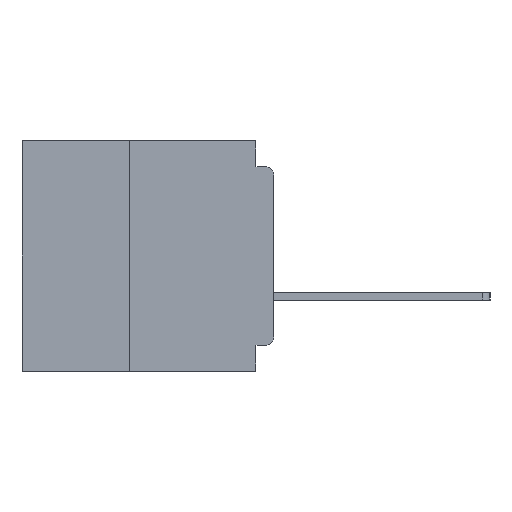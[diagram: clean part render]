
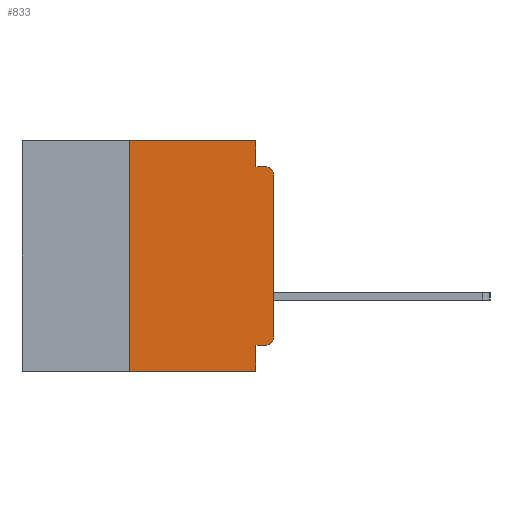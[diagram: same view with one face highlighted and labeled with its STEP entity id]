
A CAD part, left-side view. The second image highlights one B-rep face of the part: STEP entity #833.
In plain terms, the highlighted planar face has unit normal (-1, 0, 0).
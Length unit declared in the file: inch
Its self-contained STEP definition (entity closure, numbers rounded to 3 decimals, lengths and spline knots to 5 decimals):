
#833 = ADVANCED_FACE ( 'NONE', ( #34483 ), #24747, .F. ) ;
#1700 = CARTESIAN_POINT ( 'NONE',  ( 0., 0.25, -0.4 ) ) ;
#1888 = AXIS2_PLACEMENT_3D ( 'NONE', #8199, #30971, #11540 ) ;
#2004 = DIRECTION ( 'NONE',  ( 0., 0., -1. ) ) ;
#3078 = VECTOR ( 'NONE', #28970, 39.37008 ) ;
#3546 = CARTESIAN_POINT ( 'NONE',  ( 0., 0.031, -0.045 ) ) ;
#4341 = EDGE_CURVE ( 'NONE', #12091, #6310, #36215, .T. ) ;
#4519 = AXIS2_PLACEMENT_3D ( 'NONE', #5737, #12362, #33074 ) ;
#4864 = CARTESIAN_POINT ( 'NONE',  ( 0., 0.437, -0.4 ) ) ;
#5737 = CARTESIAN_POINT ( 'NONE',  ( 0., 0.437, 0. ) ) ;
#6036 = LINE ( 'NONE', #22973, #40578 ) ;
#6056 = CARTESIAN_POINT ( 'NONE',  ( 0., 0.437, 0. ) ) ;
#6310 = VERTEX_POINT ( 'NONE', #41696 ) ;
#6541 = DIRECTION ( 'NONE',  ( 0., 0., 1. ) ) ;
#7229 = CARTESIAN_POINT ( 'NONE',  ( 0., 0., -0.06 ) ) ;
#7596 = ORIENTED_EDGE ( 'NONE', *, *, #29237, .F. ) ;
#7837 = CARTESIAN_POINT ( 'NONE',  ( 0., 0.015, -0.045 ) ) ;
#8014 = VERTEX_POINT ( 'NONE', #34835 ) ;
#8199 = CARTESIAN_POINT ( 'NONE',  ( 0., 0.015, -0.06 ) ) ;
#8416 = VERTEX_POINT ( 'NONE', #7837 ) ;
#8813 = EDGE_LOOP ( 'NONE', ( #40553, #31541, #15379, #7596, #10747, #30078, #39593, #16959, #27591, #11272 ) ) ;
#10429 = DIRECTION ( 'NONE',  ( 0., 0., -1. ) ) ;
#10747 = ORIENTED_EDGE ( 'NONE', *, *, #38561, .F. ) ;
#11272 = ORIENTED_EDGE ( 'NONE', *, *, #4341, .T. ) ;
#11540 = DIRECTION ( 'NONE',  ( 0., 0., -1. ) ) ;
#12091 = VERTEX_POINT ( 'NONE', #33267 ) ;
#12362 = DIRECTION ( 'NONE',  ( 1., 0., 0. ) ) ;
#12911 = LINE ( 'NONE', #27486, #37669 ) ;
#13621 = CARTESIAN_POINT ( 'NONE',  ( 0., 0., 0. ) ) ;
#13767 = LINE ( 'NONE', #41683, #38481 ) ;
#13808 = EDGE_CURVE ( 'NONE', #6310, #17560, #40300, .T. ) ;
#15379 = ORIENTED_EDGE ( 'NONE', *, *, #31614, .F. ) ;
#15639 = VECTOR ( 'NONE', #36206, 39.37008 ) ;
#16448 = CARTESIAN_POINT ( 'NONE',  ( 0., 0.031, 0. ) ) ;
#16959 = ORIENTED_EDGE ( 'NONE', *, *, #30314, .F. ) ;
#17166 = CIRCLE ( 'NONE', #1888, 0.015 ) ;
#17560 = VERTEX_POINT ( 'NONE', #7229 ) ;
#19021 = AXIS2_PLACEMENT_3D ( 'NONE', #40917, #21693, #2004 ) ;
#19608 = LINE ( 'NONE', #6056, #3078 ) ;
#20129 = VERTEX_POINT ( 'NONE', #1700 ) ;
#20197 = CARTESIAN_POINT ( 'NONE',  ( 0., 0.031, -0.4 ) ) ;
#21693 = DIRECTION ( 'NONE',  ( -1., 0., 0. ) ) ;
#22025 = VECTOR ( 'NONE', #10429, 39.37008 ) ;
#22428 = EDGE_CURVE ( 'NONE', #12091, #37332, #13767, .T. ) ;
#22973 = CARTESIAN_POINT ( 'NONE',  ( 0., 0.25, -0.4 ) ) ;
#23073 = LINE ( 'NONE', #20197, #22025 ) ;
#23334 = DIRECTION ( 'NONE',  ( 0., -1., 0. ) ) ;
#23534 = VECTOR ( 'NONE', #24587, 39.37008 ) ;
#23976 = VECTOR ( 'NONE', #23334, 39.37008 ) ;
#24188 = VERTEX_POINT ( 'NONE', #40174 ) ;
#24547 = LINE ( 'NONE', #4864, #23534 ) ;
#24587 = DIRECTION ( 'NONE',  ( 0., -1., 0. ) ) ;
#24747 = PLANE ( 'NONE',  #4519 ) ;
#25371 = EDGE_CURVE ( 'NONE', #17560, #8416, #17166, .T. ) ;
#25845 = CARTESIAN_POINT ( 'NONE',  ( 0., 0.031, -0.355 ) ) ;
#27486 = CARTESIAN_POINT ( 'NONE',  ( 0., 0.031, 0. ) ) ;
#27591 = ORIENTED_EDGE ( 'NONE', *, *, #22428, .F. ) ;
#28228 = VERTEX_POINT ( 'NONE', #3546 ) ;
#28970 = DIRECTION ( 'NONE',  ( 0., -1., 0. ) ) ;
#29237 = EDGE_CURVE ( 'NONE', #39258, #28228, #12911, .T. ) ;
#30078 = ORIENTED_EDGE ( 'NONE', *, *, #39760, .F. ) ;
#30314 = EDGE_CURVE ( 'NONE', #37332, #8014, #23073, .T. ) ;
#30971 = DIRECTION ( 'NONE',  ( -1., 0., 0. ) ) ;
#31541 = ORIENTED_EDGE ( 'NONE', *, *, #25371, .T. ) ;
#31614 = EDGE_CURVE ( 'NONE', #28228, #8416, #37948, .T. ) ;
#33074 = DIRECTION ( 'NONE',  ( 0., 0., -1. ) ) ;
#33267 = CARTESIAN_POINT ( 'NONE',  ( 0., 0.015, -0.355 ) ) ;
#34483 = FACE_OUTER_BOUND ( 'NONE', #8813, .T. ) ;
#34835 = CARTESIAN_POINT ( 'NONE',  ( 0., 0.031, -0.4 ) ) ;
#36206 = DIRECTION ( 'NONE',  ( 0., 0., 1. ) ) ;
#36215 = CIRCLE ( 'NONE', #19021, 0.015 ) ;
#37332 = VERTEX_POINT ( 'NONE', #25845 ) ;
#37669 = VECTOR ( 'NONE', #40331, 39.37008 ) ;
#37948 = LINE ( 'NONE', #39272, #23976 ) ;
#38467 = DIRECTION ( 'NONE',  ( 0., 1., 0. ) ) ;
#38481 = VECTOR ( 'NONE', #38467, 39.37008 ) ;
#38561 = EDGE_CURVE ( 'NONE', #24188, #39258, #19608, .T. ) ;
#39258 = VERTEX_POINT ( 'NONE', #16448 ) ;
#39272 = CARTESIAN_POINT ( 'NONE',  ( 0., 0., -0.045 ) ) ;
#39593 = ORIENTED_EDGE ( 'NONE', *, *, #40139, .T. ) ;
#39760 = EDGE_CURVE ( 'NONE', #20129, #24188, #6036, .T. ) ;
#40139 = EDGE_CURVE ( 'NONE', #20129, #8014, #24547, .T. ) ;
#40174 = CARTESIAN_POINT ( 'NONE',  ( 0., 0.25, 0. ) ) ;
#40300 = LINE ( 'NONE', #13621, #15639 ) ;
#40331 = DIRECTION ( 'NONE',  ( 0., 0., -1. ) ) ;
#40553 = ORIENTED_EDGE ( 'NONE', *, *, #13808, .T. ) ;
#40578 = VECTOR ( 'NONE', #6541, 39.37008 ) ;
#40917 = CARTESIAN_POINT ( 'NONE',  ( 0., 0.015, -0.34 ) ) ;
#41683 = CARTESIAN_POINT ( 'NONE',  ( 0., 0., -0.355 ) ) ;
#41696 = CARTESIAN_POINT ( 'NONE',  ( 0., 0., -0.34 ) ) ;
